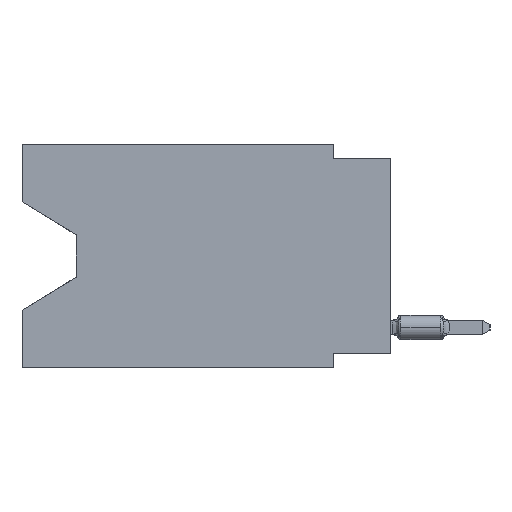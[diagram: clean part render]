
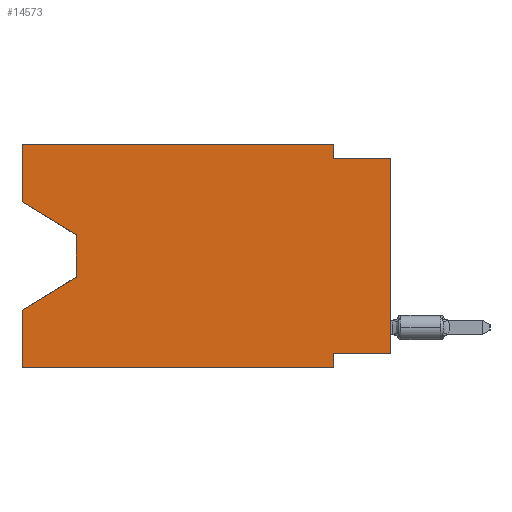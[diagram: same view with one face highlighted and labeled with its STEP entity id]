
A CAD part, left-side view. The second image highlights one B-rep face of the part: STEP entity #14573.
In plain terms, the highlighted planar face has unit normal (-1, 0, 0).
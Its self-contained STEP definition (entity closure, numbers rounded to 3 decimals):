
#101 = CARTESIAN_POINT ( 'NONE',  ( 0., 16.383, -9.906 ) ) ;
#266 = DIRECTION ( 'NONE',  ( 0., 0., -1. ) ) ;
#597 = EDGE_CURVE ( 'NONE', #15672, #5598, #6805, .T. ) ;
#846 = DIRECTION ( 'NONE',  ( 0., 0., 1. ) ) ;
#1191 = LINE ( 'NONE', #17324, #13566 ) ;
#1267 = ORIENTED_EDGE ( 'NONE', *, *, #22598, .F. ) ;
#1527 = EDGE_CURVE ( 'NONE', #5598, #22552, #15070, .T. ) ;
#1532 = DIRECTION ( 'NONE',  ( 0., 0., -1. ) ) ;
#2013 = VECTOR ( 'NONE', #22397, 1000. ) ;
#2297 = ORIENTED_EDGE ( 'NONE', *, *, #22927, .T. ) ;
#2333 = CARTESIAN_POINT ( 'NONE',  ( 0., 13.97, -5.893 ) ) ;
#2582 = VECTOR ( 'NONE', #1532, 1000. ) ;
#3144 = DIRECTION ( 'NONE',  ( 0., -0.855, -0.519 ) ) ;
#3753 = VERTEX_POINT ( 'NONE', #6192 ) ;
#4036 = CARTESIAN_POINT ( 'NONE',  ( 0., 16.383, -7.36 ) ) ;
#4066 = DIRECTION ( 'NONE',  ( 0., -1., 0. ) ) ;
#5287 = DIRECTION ( 'NONE',  ( 1., 0., 0. ) ) ;
#5297 = LINE ( 'NONE', #12769, #23479 ) ;
#5346 = LINE ( 'NONE', #14600, #7879 ) ;
#5363 = CARTESIAN_POINT ( 'NONE',  ( 0., 16.383, -9.906 ) ) ;
#5598 = VERTEX_POINT ( 'NONE', #17334 ) ;
#5669 = DIRECTION ( 'NONE',  ( 0., -1., 0. ) ) ;
#5851 = CARTESIAN_POINT ( 'NONE',  ( 0., 2.54, -9.906 ) ) ;
#6192 = CARTESIAN_POINT ( 'NONE',  ( 0., 0., -9.271 ) ) ;
#6282 = CARTESIAN_POINT ( 'NONE',  ( 0., 13.97, -4.013 ) ) ;
#6663 = VECTOR ( 'NONE', #266, 1000. ) ;
#6716 = VERTEX_POINT ( 'NONE', #10902 ) ;
#6805 = LINE ( 'NONE', #21464, #14052 ) ;
#7065 = CARTESIAN_POINT ( 'NONE',  ( 0., 2.54, -9.906 ) ) ;
#7587 = ORIENTED_EDGE ( 'NONE', *, *, #20760, .F. ) ;
#7600 = CARTESIAN_POINT ( 'NONE',  ( 0., 0., -0.635 ) ) ;
#7795 = LINE ( 'NONE', #101, #12465 ) ;
#7879 = VECTOR ( 'NONE', #10679, 1000. ) ;
#8369 = DIRECTION ( 'NONE',  ( 0., 0., -1. ) ) ;
#8538 = ORIENTED_EDGE ( 'NONE', *, *, #22154, .T. ) ;
#8811 = ORIENTED_EDGE ( 'NONE', *, *, #15551, .F. ) ;
#8828 = CARTESIAN_POINT ( 'NONE',  ( 0., 16.383, 0. ) ) ;
#8973 = EDGE_CURVE ( 'NONE', #3753, #11181, #5346, .T. ) ;
#9188 = VECTOR ( 'NONE', #20358, 1000. ) ;
#9201 = CARTESIAN_POINT ( 'NONE',  ( 0., 16.383, 0. ) ) ;
#10121 = VECTOR ( 'NONE', #5669, 1000. ) ;
#10221 = ORIENTED_EDGE ( 'NONE', *, *, #19290, .T. ) ;
#10501 = CARTESIAN_POINT ( 'NONE',  ( 0., 2.54, 0. ) ) ;
#10679 = DIRECTION ( 'NONE',  ( 0., 1., 0. ) ) ;
#10689 = CARTESIAN_POINT ( 'NONE',  ( 0., 16.383, 0. ) ) ;
#10842 = FACE_OUTER_BOUND ( 'NONE', #17853, .T. ) ;
#10902 = CARTESIAN_POINT ( 'NONE',  ( 0., 16.383, -2.546 ) ) ;
#11181 = VERTEX_POINT ( 'NONE', #21001 ) ;
#11499 = LINE ( 'NONE', #18825, #12855 ) ;
#11666 = CARTESIAN_POINT ( 'NONE',  ( 0., 0., -0.635 ) ) ;
#11947 = VERTEX_POINT ( 'NONE', #5851 ) ;
#12465 = VECTOR ( 'NONE', #4066, 1000. ) ;
#12628 = ORIENTED_EDGE ( 'NONE', *, *, #597, .T. ) ;
#12704 = EDGE_CURVE ( 'NONE', #22449, #22552, #12931, .T. ) ;
#12769 = CARTESIAN_POINT ( 'NONE',  ( 0., 16.383, -2.546 ) ) ;
#12855 = VECTOR ( 'NONE', #20275, 1000. ) ;
#12931 = LINE ( 'NONE', #9201, #9188 ) ;
#13068 = ORIENTED_EDGE ( 'NONE', *, *, #15447, .F. ) ;
#13310 = EDGE_CURVE ( 'NONE', #11181, #11947, #21283, .T. ) ;
#13566 = VECTOR ( 'NONE', #846, 1000. ) ;
#13729 = LINE ( 'NONE', #19368, #20869 ) ;
#14013 = CARTESIAN_POINT ( 'NONE',  ( 0., 2.54, -0.635 ) ) ;
#14052 = VECTOR ( 'NONE', #8369, 1000. ) ;
#14573 = ADVANCED_FACE ( 'NONE', ( #10842 ), #18152, .F. ) ;
#14600 = CARTESIAN_POINT ( 'NONE',  ( 0., 0., -9.271 ) ) ;
#15067 = ORIENTED_EDGE ( 'NONE', *, *, #1527, .T. ) ;
#15070 = LINE ( 'NONE', #2333, #2013 ) ;
#15447 = EDGE_CURVE ( 'NONE', #23327, #18791, #16862, .T. ) ;
#15551 = EDGE_CURVE ( 'NONE', #19243, #23327, #22256, .T. ) ;
#15606 = ORIENTED_EDGE ( 'NONE', *, *, #8973, .F. ) ;
#15672 = VERTEX_POINT ( 'NONE', #6282 ) ;
#16743 = CARTESIAN_POINT ( 'NONE',  ( 0., 2.54, 0. ) ) ;
#16862 = LINE ( 'NONE', #7600, #10121 ) ;
#17324 = CARTESIAN_POINT ( 'NONE',  ( 0., 16.383, 0. ) ) ;
#17334 = CARTESIAN_POINT ( 'NONE',  ( 0., 13.97, -5.893 ) ) ;
#17853 = EDGE_LOOP ( 'NONE', ( #10221, #12628, #15067, #17944, #8538, #19714, #15606, #2297, #13068, #8811, #1267, #7587 ) ) ;
#17944 = ORIENTED_EDGE ( 'NONE', *, *, #12704, .F. ) ;
#18036 = DIRECTION ( 'NONE',  ( 0., 0., -1. ) ) ;
#18152 = PLANE ( 'NONE',  #21048 ) ;
#18791 = VERTEX_POINT ( 'NONE', #11666 ) ;
#18825 = CARTESIAN_POINT ( 'NONE',  ( 0., 16.383, 0. ) ) ;
#19243 = VERTEX_POINT ( 'NONE', #10501 ) ;
#19290 = EDGE_CURVE ( 'NONE', #6716, #15672, #5297, .T. ) ;
#19368 = CARTESIAN_POINT ( 'NONE',  ( 0., 0., 0. ) ) ;
#19714 = ORIENTED_EDGE ( 'NONE', *, *, #13310, .F. ) ;
#20275 = DIRECTION ( 'NONE',  ( 0., -1., 0. ) ) ;
#20358 = DIRECTION ( 'NONE',  ( 0., 0., 1. ) ) ;
#20760 = EDGE_CURVE ( 'NONE', #6716, #21310, #1191, .T. ) ;
#20869 = VECTOR ( 'NONE', #21046, 1000. ) ;
#21001 = CARTESIAN_POINT ( 'NONE',  ( 0., 2.54, -9.271 ) ) ;
#21046 = DIRECTION ( 'NONE',  ( 0., 0., 1. ) ) ;
#21048 = AXIS2_PLACEMENT_3D ( 'NONE', #8828, #5287, #18036 ) ;
#21283 = LINE ( 'NONE', #7065, #2582 ) ;
#21310 = VERTEX_POINT ( 'NONE', #10689 ) ;
#21464 = CARTESIAN_POINT ( 'NONE',  ( 0., 13.97, -4.013 ) ) ;
#22154 = EDGE_CURVE ( 'NONE', #22449, #11947, #7795, .T. ) ;
#22256 = LINE ( 'NONE', #16743, #6663 ) ;
#22397 = DIRECTION ( 'NONE',  ( 0., 0.855, -0.519 ) ) ;
#22449 = VERTEX_POINT ( 'NONE', #5363 ) ;
#22552 = VERTEX_POINT ( 'NONE', #4036 ) ;
#22598 = EDGE_CURVE ( 'NONE', #21310, #19243, #11499, .T. ) ;
#22927 = EDGE_CURVE ( 'NONE', #3753, #18791, #13729, .T. ) ;
#23327 = VERTEX_POINT ( 'NONE', #14013 ) ;
#23479 = VECTOR ( 'NONE', #3144, 1000. ) ;
